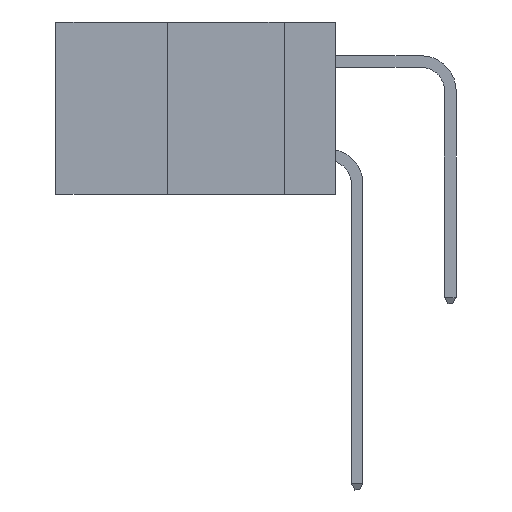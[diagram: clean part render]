
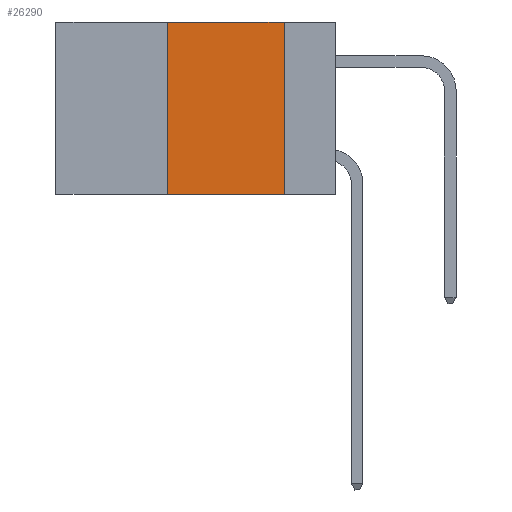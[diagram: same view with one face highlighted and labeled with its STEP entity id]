
A CAD part, left-side view. The second image highlights one B-rep face of the part: STEP entity #26290.
In plain terms, the highlighted planar face has unit normal (-1, 0, 0).
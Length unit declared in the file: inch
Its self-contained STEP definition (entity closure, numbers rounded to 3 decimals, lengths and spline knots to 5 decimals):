
#1516 = VERTEX_POINT ( 'NONE', #8686 ) ;
#1680 = DIRECTION ( 'NONE',  ( 0., -1., 0. ) ) ;
#2885 = EDGE_CURVE ( 'NONE', #4336, #1516, #18318, .T. ) ;
#3465 = FACE_OUTER_BOUND ( 'NONE', #16281, .T. ) ;
#4112 = VERTEX_POINT ( 'NONE', #24693 ) ;
#4336 = VERTEX_POINT ( 'NONE', #21879 ) ;
#6279 = DIRECTION ( 'NONE',  ( 0., -1., 0. ) ) ;
#8089 = VECTOR ( 'NONE', #24875, 39.37008 ) ;
#8392 = ORIENTED_EDGE ( 'NONE', *, *, #17561, .F. ) ;
#8686 = CARTESIAN_POINT ( 'NONE',  ( 0., 0.36, 0. ) ) ;
#8880 = DIRECTION ( 'NONE',  ( 0., 0., -1. ) ) ;
#9111 = CARTESIAN_POINT ( 'NONE',  ( 0., 0.11, -0.37 ) ) ;
#9913 = CARTESIAN_POINT ( 'NONE',  ( 0., 0.11, 0. ) ) ;
#12880 = LINE ( 'NONE', #21405, #19410 ) ;
#13127 = EDGE_CURVE ( 'NONE', #4112, #22692, #24836, .T. ) ;
#14269 = DIRECTION ( 'NONE',  ( 0., 0., -1. ) ) ;
#14871 = VECTOR ( 'NONE', #14269, 39.37008 ) ;
#14958 = CARTESIAN_POINT ( 'NONE',  ( 0., 0.6, -0.37 ) ) ;
#16281 = EDGE_LOOP ( 'NONE', ( #18180, #8392, #18219, #21151 ) ) ;
#17246 = LINE ( 'NONE', #14958, #20692 ) ;
#17561 = EDGE_CURVE ( 'NONE', #1516, #4112, #12880, .T. ) ;
#18180 = ORIENTED_EDGE ( 'NONE', *, *, #13127, .F. ) ;
#18219 = ORIENTED_EDGE ( 'NONE', *, *, #2885, .F. ) ;
#18318 = LINE ( 'NONE', #22681, #8089 ) ;
#19410 = VECTOR ( 'NONE', #1680, 39.37008 ) ;
#19490 = PLANE ( 'NONE',  #27576 ) ;
#19775 = CARTESIAN_POINT ( 'NONE',  ( 0., 0.6, 0. ) ) ;
#20692 = VECTOR ( 'NONE', #6279, 39.37008 ) ;
#21151 = ORIENTED_EDGE ( 'NONE', *, *, #21788, .T. ) ;
#21405 = CARTESIAN_POINT ( 'NONE',  ( 0., 0.6, 0. ) ) ;
#21788 = EDGE_CURVE ( 'NONE', #4336, #22692, #17246, .T. ) ;
#21879 = CARTESIAN_POINT ( 'NONE',  ( 0., 0.36, -0.37 ) ) ;
#21984 = DIRECTION ( 'NONE',  ( 1., 0., 0. ) ) ;
#22681 = CARTESIAN_POINT ( 'NONE',  ( 0., 0.36, 0. ) ) ;
#22692 = VERTEX_POINT ( 'NONE', #9111 ) ;
#24693 = CARTESIAN_POINT ( 'NONE',  ( 0., 0.11, 0. ) ) ;
#24836 = LINE ( 'NONE', #9913, #14871 ) ;
#24875 = DIRECTION ( 'NONE',  ( 0., 0., 1. ) ) ;
#26290 = ADVANCED_FACE ( 'NONE', ( #3465 ), #19490, .F. ) ;
#27576 = AXIS2_PLACEMENT_3D ( 'NONE', #19775, #21984, #8880 ) ;
